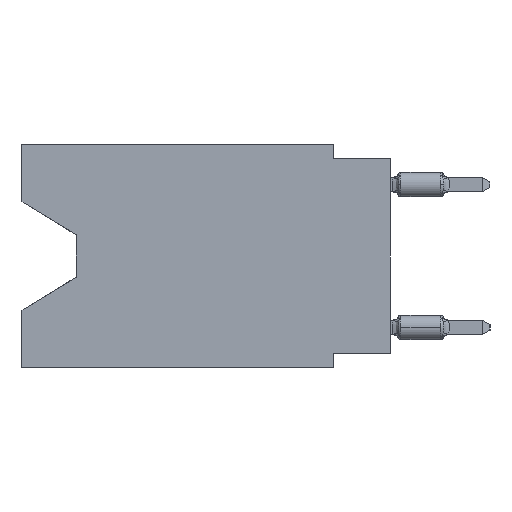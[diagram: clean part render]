
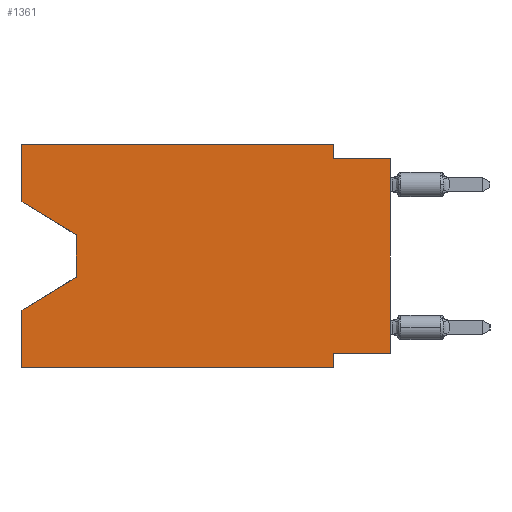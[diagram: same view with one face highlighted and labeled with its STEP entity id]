
A CAD part, left-side view. The second image highlights one B-rep face of the part: STEP entity #1361.
In plain terms, the highlighted planar face has unit normal (-1, 0, 0).
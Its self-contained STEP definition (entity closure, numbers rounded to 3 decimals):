
#362 = CARTESIAN_POINT ( 'NONE',  ( 0., 16.383, -7.36 ) ) ;
#849 = CARTESIAN_POINT ( 'NONE',  ( 0., 16.383, 0. ) ) ;
#898 = EDGE_CURVE ( 'NONE', #5079, #22406, #10544, .T. ) ;
#909 = CARTESIAN_POINT ( 'NONE',  ( 0., 13.97, -4.013 ) ) ;
#966 = VECTOR ( 'NONE', #22691, 1000. ) ;
#1103 = PLANE ( 'NONE',  #3323 ) ;
#1361 = ADVANCED_FACE ( 'NONE', ( #13806 ), #1103, .F. ) ;
#1931 = ORIENTED_EDGE ( 'NONE', *, *, #4141, .F. ) ;
#2771 = DIRECTION ( 'NONE',  ( 0., 0., 1. ) ) ;
#3028 = CARTESIAN_POINT ( 'NONE',  ( 0., 0., -0.635 ) ) ;
#3282 = LINE ( 'NONE', #13253, #15147 ) ;
#3323 = AXIS2_PLACEMENT_3D ( 'NONE', #24322, #15873, #19711 ) ;
#3537 = DIRECTION ( 'NONE',  ( 0., 0., -1. ) ) ;
#4141 = EDGE_CURVE ( 'NONE', #22852, #16047, #23935, .T. ) ;
#4245 = CARTESIAN_POINT ( 'NONE',  ( 0., 16.383, 0. ) ) ;
#4293 = CARTESIAN_POINT ( 'NONE',  ( 0., 13.97, -4.013 ) ) ;
#4608 = EDGE_CURVE ( 'NONE', #22852, #12858, #11827, .T. ) ;
#4929 = DIRECTION ( 'NONE',  ( 0., 0., 1. ) ) ;
#5079 = VERTEX_POINT ( 'NONE', #22333 ) ;
#5197 = LINE ( 'NONE', #15729, #10900 ) ;
#5689 = ORIENTED_EDGE ( 'NONE', *, *, #23325, .T. ) ;
#6244 = CARTESIAN_POINT ( 'NONE',  ( 0., 2.54, -9.906 ) ) ;
#6746 = LINE ( 'NONE', #7150, #15317 ) ;
#7125 = ORIENTED_EDGE ( 'NONE', *, *, #898, .F. ) ;
#7150 = CARTESIAN_POINT ( 'NONE',  ( 0., 0., -9.271 ) ) ;
#7252 = DIRECTION ( 'NONE',  ( 0., 0.855, -0.519 ) ) ;
#7430 = LINE ( 'NONE', #11643, #7535 ) ;
#7535 = VECTOR ( 'NONE', #9601, 1000. ) ;
#7606 = ORIENTED_EDGE ( 'NONE', *, *, #14169, .F. ) ;
#7743 = DIRECTION ( 'NONE',  ( 0., -0.855, -0.519 ) ) ;
#7994 = VERTEX_POINT ( 'NONE', #3028 ) ;
#8037 = CARTESIAN_POINT ( 'NONE',  ( 0., 2.54, 0. ) ) ;
#8064 = EDGE_CURVE ( 'NONE', #19578, #7994, #5197, .T. ) ;
#8586 = VERTEX_POINT ( 'NONE', #14317 ) ;
#8736 = EDGE_CURVE ( 'NONE', #16284, #26328, #27004, .T. ) ;
#9601 = DIRECTION ( 'NONE',  ( 0., -1., 0. ) ) ;
#9791 = ORIENTED_EDGE ( 'NONE', *, *, #8736, .F. ) ;
#10544 = LINE ( 'NONE', #849, #15100 ) ;
#10809 = CARTESIAN_POINT ( 'NONE',  ( 0., 2.54, 0. ) ) ;
#10900 = VECTOR ( 'NONE', #4929, 1000. ) ;
#11508 = EDGE_CURVE ( 'NONE', #19901, #18487, #26621, .T. ) ;
#11601 = CARTESIAN_POINT ( 'NONE',  ( 0., 2.54, -0.635 ) ) ;
#11643 = CARTESIAN_POINT ( 'NONE',  ( 0., 0., -0.635 ) ) ;
#11700 = ORIENTED_EDGE ( 'NONE', *, *, #19605, .F. ) ;
#11746 = ORIENTED_EDGE ( 'NONE', *, *, #8064, .T. ) ;
#11827 = LINE ( 'NONE', #20193, #20912 ) ;
#12682 = VECTOR ( 'NONE', #22905, 1000. ) ;
#12858 = VERTEX_POINT ( 'NONE', #909 ) ;
#13253 = CARTESIAN_POINT ( 'NONE',  ( 0., 13.97, -5.893 ) ) ;
#13427 = DIRECTION ( 'NONE',  ( 0., 1., 0. ) ) ;
#13806 = FACE_OUTER_BOUND ( 'NONE', #15288, .T. ) ;
#14169 = EDGE_CURVE ( 'NONE', #19578, #16284, #6746, .T. ) ;
#14317 = CARTESIAN_POINT ( 'NONE',  ( 0., 13.97, -5.893 ) ) ;
#14366 = LINE ( 'NONE', #4245, #966 ) ;
#14389 = CARTESIAN_POINT ( 'NONE',  ( 0., 2.54, -9.906 ) ) ;
#14963 = CARTESIAN_POINT ( 'NONE',  ( 0., 16.383, -2.546 ) ) ;
#15100 = VECTOR ( 'NONE', #25316, 1000. ) ;
#15147 = VECTOR ( 'NONE', #7252, 1000. ) ;
#15288 = EDGE_LOOP ( 'NONE', ( #19097, #18830, #5689, #7125, #23943, #9791, #7606, #11746, #11700, #23386, #26203, #1931 ) ) ;
#15317 = VECTOR ( 'NONE', #13427, 1000. ) ;
#15729 = CARTESIAN_POINT ( 'NONE',  ( 0., 0., 0. ) ) ;
#15873 = DIRECTION ( 'NONE',  ( 1., 0., 0. ) ) ;
#16047 = VERTEX_POINT ( 'NONE', #26907 ) ;
#16284 = VERTEX_POINT ( 'NONE', #24419 ) ;
#16823 = VECTOR ( 'NONE', #3537, 1000. ) ;
#16965 = VECTOR ( 'NONE', #2771, 1000. ) ;
#16999 = VECTOR ( 'NONE', #23273, 1000. ) ;
#17365 = EDGE_CURVE ( 'NONE', #5079, #26328, #26636, .T. ) ;
#18487 = VERTEX_POINT ( 'NONE', #11601 ) ;
#18596 = EDGE_CURVE ( 'NONE', #16047, #19901, #14366, .T. ) ;
#18830 = ORIENTED_EDGE ( 'NONE', *, *, #21676, .T. ) ;
#19097 = ORIENTED_EDGE ( 'NONE', *, *, #4608, .T. ) ;
#19578 = VERTEX_POINT ( 'NONE', #25744 ) ;
#19605 = EDGE_CURVE ( 'NONE', #18487, #7994, #7430, .T. ) ;
#19711 = DIRECTION ( 'NONE',  ( 0., 0., -1. ) ) ;
#19901 = VERTEX_POINT ( 'NONE', #10809 ) ;
#20193 = CARTESIAN_POINT ( 'NONE',  ( 0., 16.383, -2.546 ) ) ;
#20912 = VECTOR ( 'NONE', #7743, 1000. ) ;
#21676 = EDGE_CURVE ( 'NONE', #12858, #8586, #22867, .T. ) ;
#22333 = CARTESIAN_POINT ( 'NONE',  ( 0., 16.383, -9.906 ) ) ;
#22406 = VERTEX_POINT ( 'NONE', #362 ) ;
#22691 = DIRECTION ( 'NONE',  ( 0., -1., 0. ) ) ;
#22852 = VERTEX_POINT ( 'NONE', #14963 ) ;
#22867 = LINE ( 'NONE', #4293, #16999 ) ;
#22905 = DIRECTION ( 'NONE',  ( 0., 0., -1. ) ) ;
#23273 = DIRECTION ( 'NONE',  ( 0., 0., -1. ) ) ;
#23325 = EDGE_CURVE ( 'NONE', #8586, #22406, #3282, .T. ) ;
#23386 = ORIENTED_EDGE ( 'NONE', *, *, #11508, .F. ) ;
#23935 = LINE ( 'NONE', #24067, #16965 ) ;
#23943 = ORIENTED_EDGE ( 'NONE', *, *, #17365, .T. ) ;
#24067 = CARTESIAN_POINT ( 'NONE',  ( 0., 16.383, 0. ) ) ;
#24322 = CARTESIAN_POINT ( 'NONE',  ( 0., 16.383, 0. ) ) ;
#24419 = CARTESIAN_POINT ( 'NONE',  ( 0., 2.54, -9.271 ) ) ;
#24583 = CARTESIAN_POINT ( 'NONE',  ( 0., 16.383, -9.906 ) ) ;
#24721 = DIRECTION ( 'NONE',  ( 0., -1., 0. ) ) ;
#25316 = DIRECTION ( 'NONE',  ( 0., 0., 1. ) ) ;
#25744 = CARTESIAN_POINT ( 'NONE',  ( 0., 0., -9.271 ) ) ;
#26203 = ORIENTED_EDGE ( 'NONE', *, *, #18596, .F. ) ;
#26212 = VECTOR ( 'NONE', #24721, 1000. ) ;
#26328 = VERTEX_POINT ( 'NONE', #14389 ) ;
#26621 = LINE ( 'NONE', #8037, #16823 ) ;
#26636 = LINE ( 'NONE', #24583, #26212 ) ;
#26907 = CARTESIAN_POINT ( 'NONE',  ( 0., 16.383, 0. ) ) ;
#27004 = LINE ( 'NONE', #6244, #12682 ) ;
